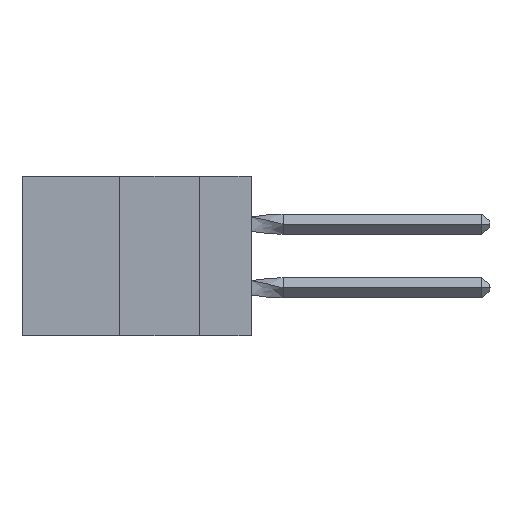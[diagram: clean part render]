
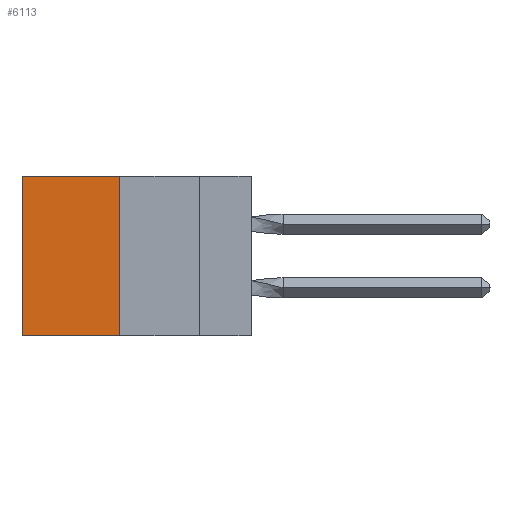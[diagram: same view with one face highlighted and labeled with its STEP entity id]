
A CAD part, left-side view. The second image highlights one B-rep face of the part: STEP entity #6113.
In plain terms, the highlighted planar face has unit normal (-1, 0, 0).
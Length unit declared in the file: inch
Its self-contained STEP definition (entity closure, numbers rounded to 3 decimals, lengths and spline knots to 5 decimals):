
#150 = CARTESIAN_POINT ( 'NONE',  ( 0.305, 0.413, -0.5 ) ) ;
#563 = FACE_OUTER_BOUND ( 'NONE', #3096, .T. ) ;
#742 = CARTESIAN_POINT ( 'NONE',  ( 0.305, 0.72, -0.5 ) ) ;
#1900 = CARTESIAN_POINT ( 'NONE',  ( 0.305, 0.413, -0.5 ) ) ;
#2291 = LINE ( 'NONE', #3540, #11375 ) ;
#2396 = VERTEX_POINT ( 'NONE', #2482 ) ;
#2482 = CARTESIAN_POINT ( 'NONE',  ( 0.305, 0.413, 0. ) ) ;
#3096 = EDGE_LOOP ( 'NONE', ( #6074, #9043, #13256, #11781 ) ) ;
#3391 = VECTOR ( 'NONE', #8888, 39.37008 ) ;
#3540 = CARTESIAN_POINT ( 'NONE',  ( 0.305, 0.72, -0.5 ) ) ;
#3860 = LINE ( 'NONE', #8177, #8212 ) ;
#4626 = DIRECTION ( 'NONE',  ( 0., 0., -1. ) ) ;
#4680 = LINE ( 'NONE', #6596, #3391 ) ;
#4701 = EDGE_CURVE ( 'NONE', #2396, #6215, #12016, .T. ) ;
#4845 = EDGE_CURVE ( 'NONE', #2396, #4941, #3860, .T. ) ;
#4941 = VERTEX_POINT ( 'NONE', #150 ) ;
#5021 = PLANE ( 'NONE',  #12625 ) ;
#5102 = VERTEX_POINT ( 'NONE', #742 ) ;
#6074 = ORIENTED_EDGE ( 'NONE', *, *, #9870, .T. ) ;
#6113 = ADVANCED_FACE ( 'NONE', ( #563 ), #5021, .F. ) ;
#6215 = VERTEX_POINT ( 'NONE', #10226 ) ;
#6596 = CARTESIAN_POINT ( 'NONE',  ( 0.305, 0.413, -0.5 ) ) ;
#8177 = CARTESIAN_POINT ( 'NONE',  ( 0.305, 0.413, -0.5 ) ) ;
#8212 = VECTOR ( 'NONE', #4626, 39.37008 ) ;
#8816 = EDGE_CURVE ( 'NONE', #4941, #5102, #4680, .T. ) ;
#8888 = DIRECTION ( 'NONE',  ( 0., 1., 0. ) ) ;
#9043 = ORIENTED_EDGE ( 'NONE', *, *, #8816, .F. ) ;
#9154 = CARTESIAN_POINT ( 'NONE',  ( 0.305, 0.413, 0. ) ) ;
#9297 = DIRECTION ( 'NONE',  ( 0., 0., -1. ) ) ;
#9870 = EDGE_CURVE ( 'NONE', #6215, #5102, #2291, .T. ) ;
#10226 = CARTESIAN_POINT ( 'NONE',  ( 0.305, 0.72, 0. ) ) ;
#10249 = DIRECTION ( 'NONE',  ( 0., 1., 0. ) ) ;
#10762 = VECTOR ( 'NONE', #10249, 39.37008 ) ;
#11375 = VECTOR ( 'NONE', #9297, 39.37008 ) ;
#11781 = ORIENTED_EDGE ( 'NONE', *, *, #4701, .T. ) ;
#12016 = LINE ( 'NONE', #9154, #10762 ) ;
#12238 = DIRECTION ( 'NONE',  ( 1., 0., 0. ) ) ;
#12625 = AXIS2_PLACEMENT_3D ( 'NONE', #1900, #12238, #13414 ) ;
#13256 = ORIENTED_EDGE ( 'NONE', *, *, #4845, .F. ) ;
#13414 = DIRECTION ( 'NONE',  ( 0., 0., -1. ) ) ;
